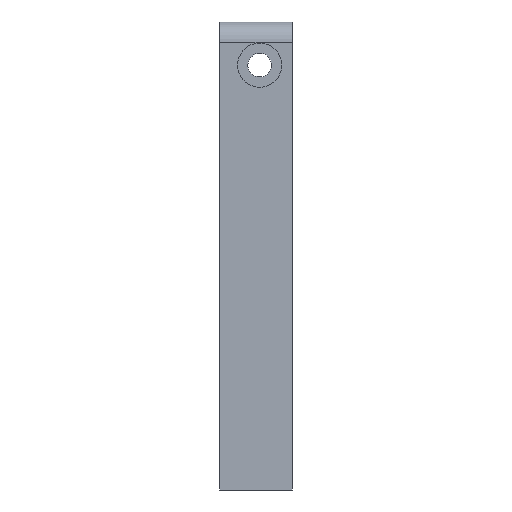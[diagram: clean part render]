
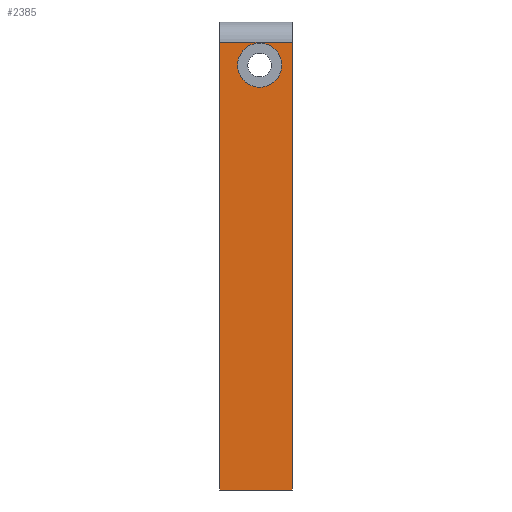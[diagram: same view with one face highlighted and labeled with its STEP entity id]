
A CAD part, front view. The second image highlights one B-rep face of the part: STEP entity #2385.
In plain terms, the highlighted planar face has unit normal (0, -1, 0).
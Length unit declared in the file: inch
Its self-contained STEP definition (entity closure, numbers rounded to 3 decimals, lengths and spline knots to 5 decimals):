
#20=FACE_BOUND('',#309,.T.);
#35=PLANE('',#2528);
#176=FACE_OUTER_BOUND('',#308,.T.);
#308=EDGE_LOOP('',(#2094,#2095,#2096,#2097));
#309=EDGE_LOOP('',(#2098));
#352=CIRCLE('',#2529,0.11024);
#664=LINE('',#8341,#772);
#687=LINE('',#8414,#795);
#688=LINE('',#8416,#796);
#689=LINE('',#8417,#797);
#772=VECTOR('',#2808,0.3937);
#795=VECTOR('',#2873,0.3937);
#796=VECTOR('',#2874,0.3937);
#797=VECTOR('',#2875,0.3937);
#1030=VERTEX_POINT('',#8338);
#1031=VERTEX_POINT('',#8340);
#1050=VERTEX_POINT('',#8413);
#1051=VERTEX_POINT('',#8415);
#1052=VERTEX_POINT('',#8418);
#1380=EDGE_CURVE('',#1031,#1030,#664,.T.);
#1412=EDGE_CURVE('',#1050,#1030,#687,.T.);
#1413=EDGE_CURVE('',#1050,#1051,#688,.T.);
#1414=EDGE_CURVE('',#1031,#1051,#689,.T.);
#1415=EDGE_CURVE('',#1052,#1052,#352,.T.);
#2094=ORIENTED_EDGE('',*,*,#1380,.T.);
#2095=ORIENTED_EDGE('',*,*,#1412,.F.);
#2096=ORIENTED_EDGE('',*,*,#1413,.T.);
#2097=ORIENTED_EDGE('',*,*,#1414,.F.);
#2098=ORIENTED_EDGE('',*,*,#1415,.T.);
#2385=ADVANCED_FACE('',(#176,#20),#35,.T.);
#2528=AXIS2_PLACEMENT_3D('',#8412,#2871,#2872);
#2529=AXIS2_PLACEMENT_3D('',#8419,#2876,#2877);
#2808=DIRECTION('',(0.,0.,-1.));
#2871=DIRECTION('center_axis',(0.,-1.,0.));
#2872=DIRECTION('ref_axis',(0.,0.,1.));
#2873=DIRECTION('',(-1.,0.,0.));
#2874=DIRECTION('',(0.,0.,1.));
#2875=DIRECTION('',(1.,0.,0.));
#2876=DIRECTION('center_axis',(0.,1.,0.));
#2877=DIRECTION('ref_axis',(1.,0.,0.));
#8338=CARTESIAN_POINT('',(0.,-2.595,-1.938));
#8340=CARTESIAN_POINT('',(0.,-2.595,0.295));
#8341=CARTESIAN_POINT('',(0.,-2.595,-1.35475));
#8412=CARTESIAN_POINT('Origin',(0.,-2.595,-1.938));
#8413=CARTESIAN_POINT('',(0.363,-2.595,-1.938));
#8414=CARTESIAN_POINT('',(0.,-2.595,-1.938));
#8415=CARTESIAN_POINT('',(0.363,-2.595,0.295));
#8416=CARTESIAN_POINT('',(0.363,-2.595,-0.25075));
#8417=CARTESIAN_POINT('',(0.105,-2.595,0.295));
#8418=CARTESIAN_POINT('',(0.08976,-2.595,0.18));
#8419=CARTESIAN_POINT('Origin',(0.2,-2.595,0.18));
